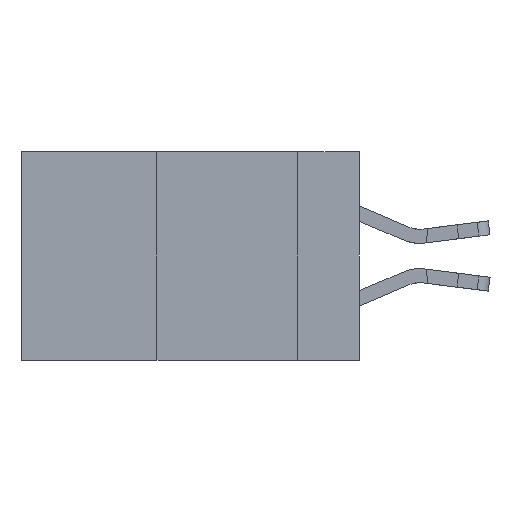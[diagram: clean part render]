
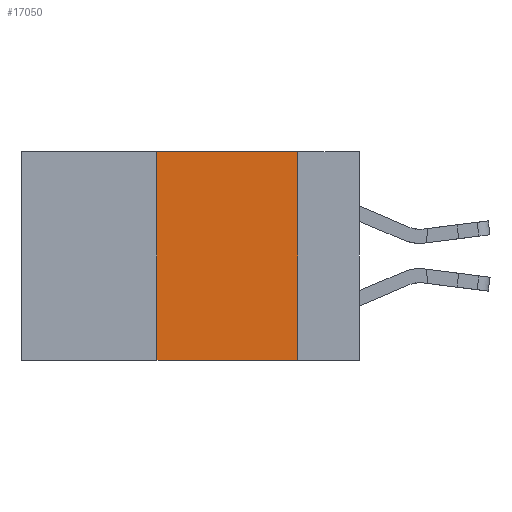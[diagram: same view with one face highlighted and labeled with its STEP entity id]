
A CAD part, left-side view. The second image highlights one B-rep face of the part: STEP entity #17050.
In plain terms, the highlighted planar face has unit normal (-1, 0, 0).
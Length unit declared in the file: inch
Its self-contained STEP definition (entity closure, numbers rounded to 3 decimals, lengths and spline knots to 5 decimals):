
#626 = CARTESIAN_POINT ( 'NONE',  ( 0., 0.36, 0. ) ) ;
#1202 = DIRECTION ( 'NONE',  ( 0., -1., 0. ) ) ;
#3604 = CARTESIAN_POINT ( 'NONE',  ( 0., 0.6, 0. ) ) ;
#6151 = DIRECTION ( 'NONE',  ( 0., -1., 0. ) ) ;
#6465 = ORIENTED_EDGE ( 'NONE', *, *, #11325, .F. ) ;
#6739 = EDGE_CURVE ( 'NONE', #29126, #9764, #16581, .T. ) ;
#7785 = DIRECTION ( 'NONE',  ( 0., 0., 1. ) ) ;
#7861 = VERTEX_POINT ( 'NONE', #16501 ) ;
#8660 = CARTESIAN_POINT ( 'NONE',  ( 0., 0.36, -0.37 ) ) ;
#9091 = LINE ( 'NONE', #10677, #16599 ) ;
#9764 = VERTEX_POINT ( 'NONE', #23504 ) ;
#10677 = CARTESIAN_POINT ( 'NONE',  ( 0., 0.6, -0.37 ) ) ;
#11267 = VECTOR ( 'NONE', #7785, 39.37008 ) ;
#11325 = EDGE_CURVE ( 'NONE', #7861, #28899, #13864, .T. ) ;
#12652 = FACE_OUTER_BOUND ( 'NONE', #22833, .T. ) ;
#13733 = EDGE_CURVE ( 'NONE', #9764, #7861, #13910, .T. ) ;
#13864 = LINE ( 'NONE', #24532, #28459 ) ;
#13910 = LINE ( 'NONE', #17116, #27792 ) ;
#14356 = ORIENTED_EDGE ( 'NONE', *, *, #6739, .F. ) ;
#14679 = DIRECTION ( 'NONE',  ( 1., 0., 0. ) ) ;
#14982 = DIRECTION ( 'NONE',  ( 0., 0., -1. ) ) ;
#15131 = DIRECTION ( 'NONE',  ( 0., 0., -1. ) ) ;
#16501 = CARTESIAN_POINT ( 'NONE',  ( 0., 0.11, 0. ) ) ;
#16581 = LINE ( 'NONE', #626, #11267 ) ;
#16582 = EDGE_CURVE ( 'NONE', #29126, #28899, #9091, .T. ) ;
#16599 = VECTOR ( 'NONE', #1202, 39.37008 ) ;
#17050 = ADVANCED_FACE ( 'NONE', ( #12652 ), #21618, .F. ) ;
#17116 = CARTESIAN_POINT ( 'NONE',  ( 0., 0.6, 0. ) ) ;
#17169 = CARTESIAN_POINT ( 'NONE',  ( 0., 0.11, -0.37 ) ) ;
#21618 = PLANE ( 'NONE',  #28919 ) ;
#22200 = ORIENTED_EDGE ( 'NONE', *, *, #16582, .T. ) ;
#22833 = EDGE_LOOP ( 'NONE', ( #6465, #26826, #14356, #22200 ) ) ;
#23504 = CARTESIAN_POINT ( 'NONE',  ( 0., 0.36, 0. ) ) ;
#24532 = CARTESIAN_POINT ( 'NONE',  ( 0., 0.11, 0. ) ) ;
#26826 = ORIENTED_EDGE ( 'NONE', *, *, #13733, .F. ) ;
#27792 = VECTOR ( 'NONE', #6151, 39.37008 ) ;
#28459 = VECTOR ( 'NONE', #15131, 39.37008 ) ;
#28899 = VERTEX_POINT ( 'NONE', #17169 ) ;
#28919 = AXIS2_PLACEMENT_3D ( 'NONE', #3604, #14679, #14982 ) ;
#29126 = VERTEX_POINT ( 'NONE', #8660 ) ;
